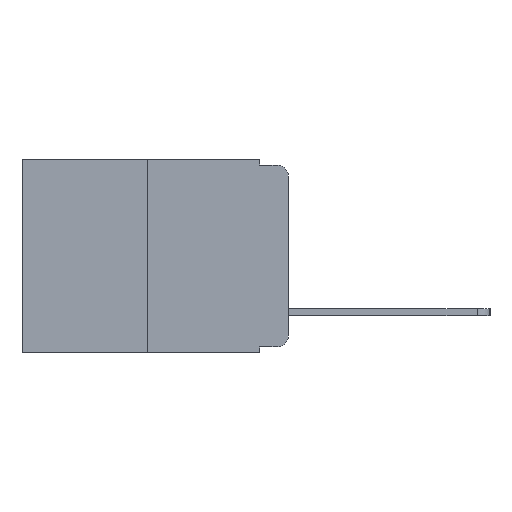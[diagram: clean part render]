
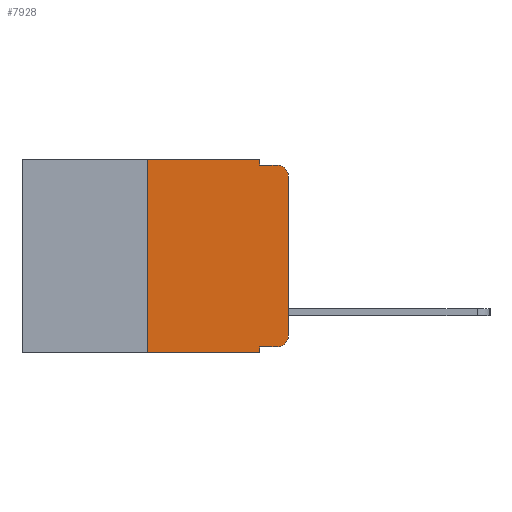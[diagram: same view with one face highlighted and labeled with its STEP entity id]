
A CAD part, left-side view. The second image highlights one B-rep face of the part: STEP entity #7928.
In plain terms, the highlighted planar face has unit normal (-1, 0, 0).
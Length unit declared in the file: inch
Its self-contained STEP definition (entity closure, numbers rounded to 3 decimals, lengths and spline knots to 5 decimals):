
#719 = EDGE_CURVE ( 'NONE', #9078, #5935, #14367, .T. ) ;
#775 = EDGE_CURVE ( 'NONE', #5935, #5809, #12723, .T. ) ;
#918 = AXIS2_PLACEMENT_3D ( 'NONE', #16389, #17189, #17165 ) ;
#929 = EDGE_CURVE ( 'NONE', #5809, #8408, #1214, .T. ) ;
#1214 = CIRCLE ( 'NONE', #918, 0.02 ) ;
#1288 = LINE ( 'NONE', #11061, #8213 ) ;
#1521 = EDGE_CURVE ( 'NONE', #10250, #15438, #4217, .T. ) ;
#1606 = VECTOR ( 'NONE', #16874, 39.37008 ) ;
#1802 = EDGE_CURVE ( 'NONE', #3050, #9369, #14263, .T. ) ;
#2046 = ORIENTED_EDGE ( 'NONE', *, *, #1802, .F. ) ;
#2114 = VECTOR ( 'NONE', #2533, 39.37008 ) ;
#2425 = ORIENTED_EDGE ( 'NONE', *, *, #929, .T. ) ;
#2468 = ORIENTED_EDGE ( 'NONE', *, *, #16189, .F. ) ;
#2533 = DIRECTION ( 'NONE',  ( 0., -1., 0. ) ) ;
#3050 = VERTEX_POINT ( 'NONE', #8453 ) ;
#3452 = CARTESIAN_POINT ( 'NONE',  ( 0., 0.473, 0. ) ) ;
#3466 = AXIS2_PLACEMENT_3D ( 'NONE', #3452, #12909, #4855 ) ;
#3702 = VERTEX_POINT ( 'NONE', #16723 ) ;
#3744 = ORIENTED_EDGE ( 'NONE', *, *, #3899, .F. ) ;
#3899 = EDGE_CURVE ( 'NONE', #3702, #9685, #11812, .T. ) ;
#3947 = DIRECTION ( 'NONE',  ( 0., 0., 1. ) ) ;
#4217 = LINE ( 'NONE', #9087, #11489 ) ;
#4460 = FACE_OUTER_BOUND ( 'NONE', #11014, .T. ) ;
#4840 = ORIENTED_EDGE ( 'NONE', *, *, #719, .T. ) ;
#4852 = EDGE_CURVE ( 'NONE', #3050, #15438, #1288, .T. ) ;
#4855 = DIRECTION ( 'NONE',  ( 0., 0., -1. ) ) ;
#5236 = CARTESIAN_POINT ( 'NONE',  ( 0., 0.051, -0.01 ) ) ;
#5260 = CARTESIAN_POINT ( 'NONE',  ( 0., 0.25, 0. ) ) ;
#5571 = VECTOR ( 'NONE', #11671, 39.37008 ) ;
#5653 = ORIENTED_EDGE ( 'NONE', *, *, #16413, .F. ) ;
#5809 = VERTEX_POINT ( 'NONE', #13687 ) ;
#5815 = CARTESIAN_POINT ( 'NONE',  ( 0., 0.051, -0.343 ) ) ;
#5935 = VERTEX_POINT ( 'NONE', #16718 ) ;
#6102 = ORIENTED_EDGE ( 'NONE', *, *, #775, .T. ) ;
#7750 = CARTESIAN_POINT ( 'NONE',  ( 0., 0.051, -0.333 ) ) ;
#7783 = CARTESIAN_POINT ( 'NONE',  ( 0., 0.02, -0.313 ) ) ;
#7928 = ADVANCED_FACE ( 'NONE', ( #4460 ), #11640, .F. ) ;
#7985 = DIRECTION ( 'NONE',  ( 0., 0., 1. ) ) ;
#7998 = DIRECTION ( 'NONE',  ( 0., 0., -1. ) ) ;
#8213 = VECTOR ( 'NONE', #10617, 39.37008 ) ;
#8408 = VERTEX_POINT ( 'NONE', #8814 ) ;
#8453 = CARTESIAN_POINT ( 'NONE',  ( 0., 0.25, -0.343 ) ) ;
#8809 = VECTOR ( 'NONE', #7985, 39.37008 ) ;
#8814 = CARTESIAN_POINT ( 'NONE',  ( 0., 0.02, -0.01 ) ) ;
#8876 = DIRECTION ( 'NONE',  ( 0., 0., -1. ) ) ;
#8959 = ORIENTED_EDGE ( 'NONE', *, *, #1521, .F. ) ;
#9078 = VERTEX_POINT ( 'NONE', #10103 ) ;
#9087 = CARTESIAN_POINT ( 'NONE',  ( 0., 0.051, 0. ) ) ;
#9171 = DIRECTION ( 'NONE',  ( 0., 0., -1. ) ) ;
#9235 = EDGE_CURVE ( 'NONE', #10250, #9078, #15460, .T. ) ;
#9369 = VERTEX_POINT ( 'NONE', #5260 ) ;
#9434 = LINE ( 'NONE', #5236, #2114 ) ;
#9685 = VERTEX_POINT ( 'NONE', #13898 ) ;
#10103 = CARTESIAN_POINT ( 'NONE',  ( 0., 0.02, -0.333 ) ) ;
#10250 = VERTEX_POINT ( 'NONE', #16233 ) ;
#10371 = CARTESIAN_POINT ( 'NONE',  ( 0., 0.473, 0. ) ) ;
#10617 = DIRECTION ( 'NONE',  ( 0., -1., 0. ) ) ;
#10872 = VECTOR ( 'NONE', #3947, 39.37008 ) ;
#11006 = VECTOR ( 'NONE', #7998, 39.37008 ) ;
#11014 = EDGE_LOOP ( 'NONE', ( #6102, #2425, #5653, #3744, #2468, #2046, #12448, #8959, #12050, #4840 ) ) ;
#11061 = CARTESIAN_POINT ( 'NONE',  ( 0., 0.473, -0.343 ) ) ;
#11489 = VECTOR ( 'NONE', #8876, 39.37008 ) ;
#11640 = PLANE ( 'NONE',  #3466 ) ;
#11671 = DIRECTION ( 'NONE',  ( 0., -1., 0. ) ) ;
#11812 = LINE ( 'NONE', #17180, #11006 ) ;
#12050 = ORIENTED_EDGE ( 'NONE', *, *, #9235, .T. ) ;
#12448 = ORIENTED_EDGE ( 'NONE', *, *, #4852, .T. ) ;
#12723 = LINE ( 'NONE', #13562, #8809 ) ;
#12909 = DIRECTION ( 'NONE',  ( 1., 0., 0. ) ) ;
#13562 = CARTESIAN_POINT ( 'NONE',  ( 0., 0., 0. ) ) ;
#13687 = CARTESIAN_POINT ( 'NONE',  ( 0., 0., -0.03 ) ) ;
#13898 = CARTESIAN_POINT ( 'NONE',  ( 0., 0.051, -0.01 ) ) ;
#14263 = LINE ( 'NONE', #15221, #10872 ) ;
#14367 = CIRCLE ( 'NONE', #15997, 0.02 ) ;
#15221 = CARTESIAN_POINT ( 'NONE',  ( 0., 0.25, 0. ) ) ;
#15438 = VERTEX_POINT ( 'NONE', #5815 ) ;
#15460 = LINE ( 'NONE', #7750, #1606 ) ;
#15997 = AXIS2_PLACEMENT_3D ( 'NONE', #7783, #16899, #9171 ) ;
#16107 = LINE ( 'NONE', #10371, #5571 ) ;
#16189 = EDGE_CURVE ( 'NONE', #9369, #3702, #16107, .T. ) ;
#16233 = CARTESIAN_POINT ( 'NONE',  ( 0., 0.051, -0.333 ) ) ;
#16389 = CARTESIAN_POINT ( 'NONE',  ( 0., 0.02, -0.03 ) ) ;
#16413 = EDGE_CURVE ( 'NONE', #9685, #8408, #9434, .T. ) ;
#16718 = CARTESIAN_POINT ( 'NONE',  ( 0., 0., -0.313 ) ) ;
#16723 = CARTESIAN_POINT ( 'NONE',  ( 0., 0.051, 0. ) ) ;
#16874 = DIRECTION ( 'NONE',  ( 0., -1., 0. ) ) ;
#16899 = DIRECTION ( 'NONE',  ( -1., 0., 0. ) ) ;
#17165 = DIRECTION ( 'NONE',  ( 0., 0., -1. ) ) ;
#17180 = CARTESIAN_POINT ( 'NONE',  ( 0., 0.051, 0. ) ) ;
#17189 = DIRECTION ( 'NONE',  ( -1., 0., 0. ) ) ;
